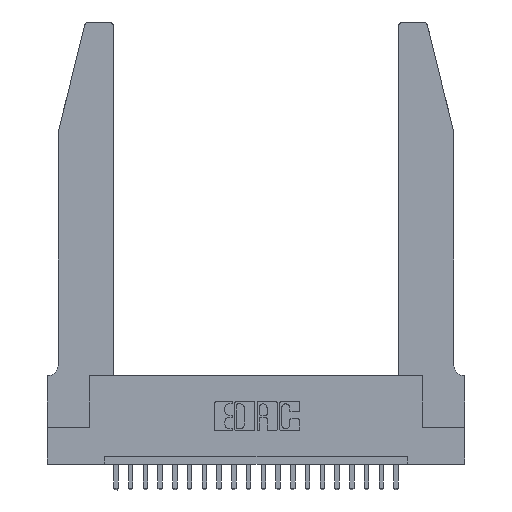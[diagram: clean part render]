
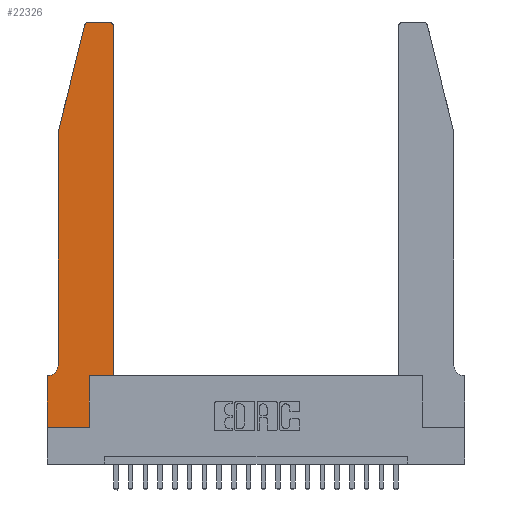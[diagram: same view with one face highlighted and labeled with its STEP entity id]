
A CAD part, top view. The second image highlights one B-rep face of the part: STEP entity #22326.
In plain terms, the highlighted planar face has unit normal (0, 0, 1).
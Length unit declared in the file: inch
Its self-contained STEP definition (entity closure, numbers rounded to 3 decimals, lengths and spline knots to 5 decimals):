
#216 = EDGE_CURVE ( 'NONE', #10877, #22018, #7928, .T. ) ;
#844 = DIRECTION ( 'NONE',  ( 1., 0., 0. ) ) ;
#900 = LINE ( 'NONE', #15012, #16417 ) ;
#1531 = CARTESIAN_POINT ( 'NONE',  ( 0., 0., 0.37 ) ) ;
#1585 = CARTESIAN_POINT ( 'NONE',  ( 0.2865, 0.35, 0.37 ) ) ;
#1882 = EDGE_CURVE ( 'NONE', #2177, #10877, #12011, .T. ) ;
#1926 = CARTESIAN_POINT ( 'NONE',  ( 0., 0.35, 0.37 ) ) ;
#2074 = VERTEX_POINT ( 'NONE', #7020 ) ;
#2177 = VERTEX_POINT ( 'NONE', #20426 ) ;
#2246 = CARTESIAN_POINT ( 'NONE',  ( 0.4505, 0.35, 0.37 ) ) ;
#2351 = DIRECTION ( 'NONE',  ( 1., 0., 0. ) ) ;
#2541 = DIRECTION ( 'NONE',  ( 0., -1., 0. ) ) ;
#2651 = VERTEX_POINT ( 'NONE', #1531 ) ;
#2716 = LINE ( 'NONE', #4433, #21222 ) ;
#2774 = VECTOR ( 'NONE', #3109, 39.37008 ) ;
#2905 = DIRECTION ( 'NONE',  ( 0., 0., -1. ) ) ;
#3109 = DIRECTION ( 'NONE',  ( 1., 0., 0. ) ) ;
#3171 = FACE_OUTER_BOUND ( 'NONE', #8154, .T. ) ;
#3424 = CARTESIAN_POINT ( 'NONE',  ( 0.0755, 2., 0.37 ) ) ;
#4433 = CARTESIAN_POINT ( 'NONE',  ( 0.0755, 0.35, 0.37 ) ) ;
#4737 = ORIENTED_EDGE ( 'NONE', *, *, #5922, .T. ) ;
#4745 = EDGE_CURVE ( 'NONE', #20836, #2177, #17136, .T. ) ;
#4783 = DIRECTION ( 'NONE',  ( -1., 0., 0. ) ) ;
#4949 = VERTEX_POINT ( 'NONE', #3424 ) ;
#4979 = CARTESIAN_POINT ( 'NONE',  ( 0.4505, 0.35, 0.37 ) ) ;
#5091 = CARTESIAN_POINT ( 'NONE',  ( 0.4205, 2.75, 0.37 ) ) ;
#5689 = DIRECTION ( 'NONE',  ( 1., 0., 0. ) ) ;
#5905 = DIRECTION ( 'NONE',  ( 1., 0., 0. ) ) ;
#5922 = EDGE_CURVE ( 'NONE', #22018, #12374, #21209, .T. ) ;
#5978 = CARTESIAN_POINT ( 'NONE',  ( 0.284, 2.72, 0.37 ) ) ;
#6136 = CARTESIAN_POINT ( 'NONE',  ( 0.2865, 0.35, 0.37 ) ) ;
#6964 = ORIENTED_EDGE ( 'NONE', *, *, #1882, .T. ) ;
#7020 = CARTESIAN_POINT ( 'NONE',  ( 0.0055, 0.35, 0.37 ) ) ;
#7296 = ORIENTED_EDGE ( 'NONE', *, *, #4745, .T. ) ;
#7928 = LINE ( 'NONE', #13719, #21425 ) ;
#8154 = EDGE_LOOP ( 'NONE', ( #22869, #4737, #9415, #11601, #19659, #8654, #10939, #18214, #15570, #20402, #7296, #6964 ) ) ;
#8173 = EDGE_CURVE ( 'NONE', #16368, #2074, #14475, .T. ) ;
#8566 = EDGE_CURVE ( 'NONE', #4949, #16368, #900, .T. ) ;
#8654 = ORIENTED_EDGE ( 'NONE', *, *, #20683, .T. ) ;
#9415 = ORIENTED_EDGE ( 'NONE', *, *, #13695, .T. ) ;
#9568 = CARTESIAN_POINT ( 'NONE',  ( 0., 0.35, 0.37 ) ) ;
#10418 = DIRECTION ( 'NONE',  ( -1., 0., 0. ) ) ;
#10691 = AXIS2_PLACEMENT_3D ( 'NONE', #9568, #12941, #5689 ) ;
#10844 = EDGE_CURVE ( 'NONE', #12257, #20517, #14749, .T. ) ;
#10877 = VERTEX_POINT ( 'NONE', #5091 ) ;
#10881 = DIRECTION ( 'NONE',  ( -0.239, -0.971, 0. ) ) ;
#10939 = ORIENTED_EDGE ( 'NONE', *, *, #13187, .T. ) ;
#11450 = DIRECTION ( 'NONE',  ( 0., -1., 0. ) ) ;
#11601 = ORIENTED_EDGE ( 'NONE', *, *, #8566, .T. ) ;
#11801 = CARTESIAN_POINT ( 'NONE',  ( 0.0055, 0.42, 0.37 ) ) ;
#12011 = CIRCLE ( 'NONE', #14487, 0.03 ) ;
#12256 = DIRECTION ( 'NONE',  ( 0., 1., 0. ) ) ;
#12257 = VERTEX_POINT ( 'NONE', #12466 ) ;
#12374 = VERTEX_POINT ( 'NONE', #12414 ) ;
#12414 = CARTESIAN_POINT ( 'NONE',  ( 0.25487, 2.72718, 0.37 ) ) ;
#12466 = CARTESIAN_POINT ( 'NONE',  ( 0.2865, 0., 0.37 ) ) ;
#12863 = PLANE ( 'NONE',  #10691 ) ;
#12941 = DIRECTION ( 'NONE',  ( 0., 0., 1. ) ) ;
#13154 = DIRECTION ( 'NONE',  ( 0., 0., 1. ) ) ;
#13187 = EDGE_CURVE ( 'NONE', #19068, #2651, #18568, .T. ) ;
#13695 = EDGE_CURVE ( 'NONE', #12374, #4949, #20171, .T. ) ;
#13719 = CARTESIAN_POINT ( 'NONE',  ( 0.2605, 2.75, 0.37 ) ) ;
#14054 = EDGE_CURVE ( 'NONE', #20517, #20836, #16314, .T. ) ;
#14076 = AXIS2_PLACEMENT_3D ( 'NONE', #5978, #18471, #2351 ) ;
#14120 = CARTESIAN_POINT ( 'NONE',  ( 0.0755, 0.42, 0.37 ) ) ;
#14462 = EDGE_CURVE ( 'NONE', #2651, #12257, #17402, .T. ) ;
#14475 = CIRCLE ( 'NONE', #17860, 0.07 ) ;
#14487 = AXIS2_PLACEMENT_3D ( 'NONE', #16866, #13154, #844 ) ;
#14655 = VECTOR ( 'NONE', #10881, 39.37008 ) ;
#14749 = LINE ( 'NONE', #1585, #17547 ) ;
#15012 = CARTESIAN_POINT ( 'NONE',  ( 0.0755, 2., 0.37 ) ) ;
#15285 = CARTESIAN_POINT ( 'NONE',  ( 0., 0., 0.37 ) ) ;
#15570 = ORIENTED_EDGE ( 'NONE', *, *, #10844, .T. ) ;
#16290 = VECTOR ( 'NONE', #5905, 39.37008 ) ;
#16314 = LINE ( 'NONE', #4979, #2774 ) ;
#16368 = VERTEX_POINT ( 'NONE', #14120 ) ;
#16417 = VECTOR ( 'NONE', #2541, 39.37008 ) ;
#16671 = CARTESIAN_POINT ( 'NONE',  ( 0., 0., 0.37 ) ) ;
#16866 = CARTESIAN_POINT ( 'NONE',  ( 0.4205, 2.72, 0.37 ) ) ;
#17136 = LINE ( 'NONE', #2246, #21544 ) ;
#17402 = LINE ( 'NONE', #15285, #16290 ) ;
#17547 = VECTOR ( 'NONE', #18988, 39.37008 ) ;
#17784 = CARTESIAN_POINT ( 'NONE',  ( 0.4505, 0.35, 0.37 ) ) ;
#17860 = AXIS2_PLACEMENT_3D ( 'NONE', #11801, #2905, #10418 ) ;
#18214 = ORIENTED_EDGE ( 'NONE', *, *, #14462, .T. ) ;
#18471 = DIRECTION ( 'NONE',  ( 0., 0., 1. ) ) ;
#18568 = LINE ( 'NONE', #16671, #22691 ) ;
#18988 = DIRECTION ( 'NONE',  ( 0., 1., 0. ) ) ;
#19068 = VERTEX_POINT ( 'NONE', #1926 ) ;
#19572 = CARTESIAN_POINT ( 'NONE',  ( 0.0755, 2., 0.37 ) ) ;
#19659 = ORIENTED_EDGE ( 'NONE', *, *, #8173, .T. ) ;
#20171 = LINE ( 'NONE', #19572, #14655 ) ;
#20394 = DIRECTION ( 'NONE',  ( -1., 0., 0. ) ) ;
#20402 = ORIENTED_EDGE ( 'NONE', *, *, #14054, .T. ) ;
#20426 = CARTESIAN_POINT ( 'NONE',  ( 0.4505, 2.72, 0.37 ) ) ;
#20517 = VERTEX_POINT ( 'NONE', #6136 ) ;
#20683 = EDGE_CURVE ( 'NONE', #2074, #19068, #2716, .T. ) ;
#20836 = VERTEX_POINT ( 'NONE', #17784 ) ;
#21103 = CARTESIAN_POINT ( 'NONE',  ( 0.284, 2.75, 0.37 ) ) ;
#21209 = CIRCLE ( 'NONE', #14076, 0.03 ) ;
#21222 = VECTOR ( 'NONE', #20394, 39.37008 ) ;
#21425 = VECTOR ( 'NONE', #4783, 39.37008 ) ;
#21544 = VECTOR ( 'NONE', #12256, 39.37008 ) ;
#22018 = VERTEX_POINT ( 'NONE', #21103 ) ;
#22326 = ADVANCED_FACE ( 'NONE', ( #3171 ), #12863, .T. ) ;
#22691 = VECTOR ( 'NONE', #11450, 39.37008 ) ;
#22869 = ORIENTED_EDGE ( 'NONE', *, *, #216, .T. ) ;
